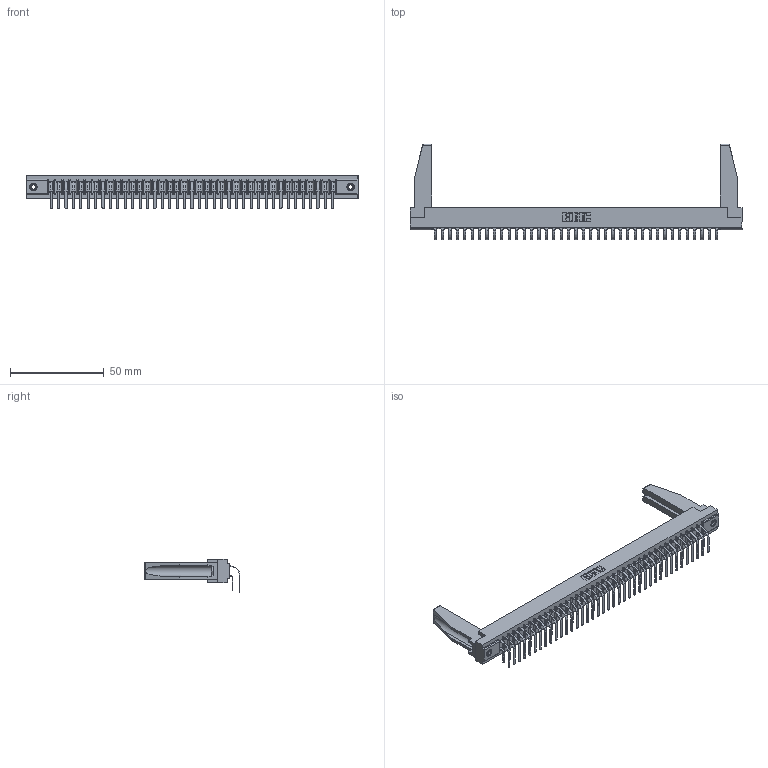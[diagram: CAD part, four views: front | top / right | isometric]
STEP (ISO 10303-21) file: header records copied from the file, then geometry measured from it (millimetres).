
FILE_DESCRIPTION (( 'STEP AP203' ), '1' );
FILE_NAME ('307-078-559-278.STEP', '2022-07-08T19:02:13', ( '' ), ( '' ), 'SwSTEP 2.0', 'SolidWorks 2020', '' );
FILE_SCHEMA (( 'CONFIG_CONTROL_DESIGN' ));
Length unit declared in the file: inch
Products named in the file (6): 307-290-001_559 - 2 (Single); 345-250-001_345-250-001-102; 307-220-078; 307-078-559-278; 307-290-001_558 559 - 1 (Single); 307 Part_.156 Dia Mounting Holes
Assembly tree (83 placements, depth 2):
  307-078-559-278
    307 Part_.156 Dia Mounting Holes
    307-290-001_558 559 - 1 (Single)  x39
    307-290-001_559 - 2 (Single)  x39
    307-220-078  x2
    345-250-001_345-250-001-102  x2
Bounding box: 177.55 x 51.22 x 18.07 mm (x, y, z)
Volume: 23145.4 mm3; surface area: 28871 mm2
Topology: 83 solids, 83 shells, 4188 faces, 11729 edges, 7598 vertices
Faces by surface type: plane 2728, cylinder 1364, sphere 80, cone 12, torus 4
Entity records: 38938 total; most frequent: CARTESIAN_POINT 6383, ORIENTED_EDGE 6284, DIRECTION 6206, EDGE_CURVE 3142, VECTOR 2412, LINE 2412, VERTEX_POINT 2032, AXIS2_PLACEMENT_3D 1897
